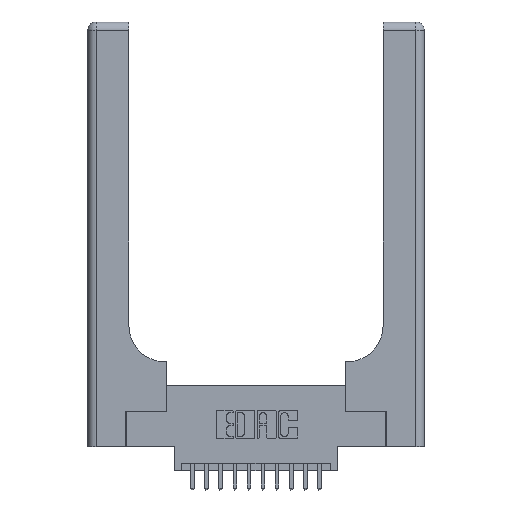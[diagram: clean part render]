
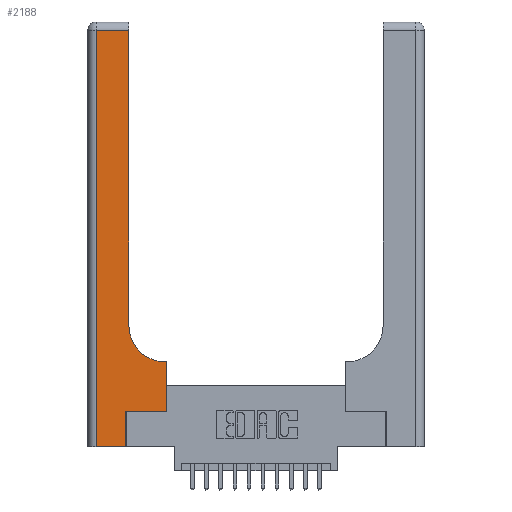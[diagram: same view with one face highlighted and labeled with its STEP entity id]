
A CAD part, top view. The second image highlights one B-rep face of the part: STEP entity #2188.
In plain terms, the highlighted planar face has unit normal (0, 0, 1).
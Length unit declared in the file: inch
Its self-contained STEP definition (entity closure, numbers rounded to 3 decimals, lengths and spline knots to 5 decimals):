
#117 = AXIS2_PLACEMENT_3D ( 'NONE', #14406, #6383, #15714 ) ;
#143 = EDGE_CURVE ( 'NONE', #3979, #8426, #5227, .T. ) ;
#165 = VERTEX_POINT ( 'NONE', #17461 ) ;
#1022 = ORIENTED_EDGE ( 'NONE', *, *, #143, .T. ) ;
#1057 = ORIENTED_EDGE ( 'NONE', *, *, #1328, .T. ) ;
#1191 = ORIENTED_EDGE ( 'NONE', *, *, #13848, .T. ) ;
#1328 = EDGE_CURVE ( 'NONE', #6525, #7529, #17280, .T. ) ;
#1577 = LINE ( 'NONE', #12074, #12004 ) ;
#1596 = CIRCLE ( 'NONE', #117, 0.25 ) ;
#1942 = EDGE_CURVE ( 'NONE', #3460, #11714, #5795, .T. ) ;
#2188 = ADVANCED_FACE ( 'NONE', ( #9169 ), #16580, .F. ) ;
#2648 = DIRECTION ( 'NONE',  ( 0., -1., 0. ) ) ;
#2666 = VERTEX_POINT ( 'NONE', #12107 ) ;
#2839 = EDGE_CURVE ( 'NONE', #2666, #165, #14156, .T. ) ;
#2860 = CARTESIAN_POINT ( 'NONE',  ( 0.06, 3., 0.37 ) ) ;
#3460 = VERTEX_POINT ( 'NONE', #4581 ) ;
#3979 = VERTEX_POINT ( 'NONE', #11305 ) ;
#3980 = CARTESIAN_POINT ( 'NONE',  ( 0.5585, 0.6, 0.37 ) ) ;
#4274 = VECTOR ( 'NONE', #10622, 39.37008 ) ;
#4581 = CARTESIAN_POINT ( 'NONE',  ( 0.2915, 0.85, 0.37 ) ) ;
#4816 = CARTESIAN_POINT ( 'NONE',  ( 0.2915, 3., 0.37 ) ) ;
#4951 = VECTOR ( 'NONE', #14915, 39.37008 ) ;
#5227 = LINE ( 'NONE', #9104, #12342 ) ;
#5795 = LINE ( 'NONE', #4816, #4951 ) ;
#5859 = EDGE_CURVE ( 'NONE', #10362, #3460, #1596, .T. ) ;
#6108 = CARTESIAN_POINT ( 'NONE',  ( 0.06, 0., 0.37 ) ) ;
#6243 = VECTOR ( 'NONE', #2648, 39.37008 ) ;
#6383 = DIRECTION ( 'NONE',  ( 0., 0., -1. ) ) ;
#6503 = LINE ( 'NONE', #16920, #16689 ) ;
#6525 = VERTEX_POINT ( 'NONE', #7737 ) ;
#6586 = LINE ( 'NONE', #15917, #7435 ) ;
#6600 = ORIENTED_EDGE ( 'NONE', *, *, #5859, .T. ) ;
#7007 = ORIENTED_EDGE ( 'NONE', *, *, #16245, .T. ) ;
#7385 = ORIENTED_EDGE ( 'NONE', *, *, #17091, .T. ) ;
#7435 = VECTOR ( 'NONE', #7964, 39.37008 ) ;
#7529 = VERTEX_POINT ( 'NONE', #6108 ) ;
#7737 = CARTESIAN_POINT ( 'NONE',  ( 0.06, 2.94, 0.37 ) ) ;
#7964 = DIRECTION ( 'NONE',  ( 1., 0., 0. ) ) ;
#8256 = ORIENTED_EDGE ( 'NONE', *, *, #1942, .T. ) ;
#8426 = VERTEX_POINT ( 'NONE', #3980 ) ;
#8581 = VECTOR ( 'NONE', #13203, 39.37008 ) ;
#8976 = DIRECTION ( 'NONE',  ( -1., 0., 0. ) ) ;
#9104 = CARTESIAN_POINT ( 'NONE',  ( 0.5585, 0.25, 0.37 ) ) ;
#9169 = FACE_OUTER_BOUND ( 'NONE', #12864, .T. ) ;
#9256 = ORIENTED_EDGE ( 'NONE', *, *, #13971, .T. ) ;
#10362 = VERTEX_POINT ( 'NONE', #13468 ) ;
#10622 = DIRECTION ( 'NONE',  ( 0., 1., 0. ) ) ;
#10803 = DIRECTION ( 'NONE',  ( -1., 0., 0. ) ) ;
#10840 = CARTESIAN_POINT ( 'NONE',  ( 0.269, 0., 0.37 ) ) ;
#11305 = CARTESIAN_POINT ( 'NONE',  ( 0.5585, 0.25, 0.37 ) ) ;
#11714 = VERTEX_POINT ( 'NONE', #13173 ) ;
#12004 = VECTOR ( 'NONE', #10803, 39.37008 ) ;
#12074 = CARTESIAN_POINT ( 'NONE',  ( 0.2915, 0.6, 0.37 ) ) ;
#12107 = CARTESIAN_POINT ( 'NONE',  ( 0.269, 0., 0.37 ) ) ;
#12342 = VECTOR ( 'NONE', #12434, 39.37008 ) ;
#12434 = DIRECTION ( 'NONE',  ( 0., 1., 0. ) ) ;
#12714 = ORIENTED_EDGE ( 'NONE', *, *, #2839, .T. ) ;
#12864 = EDGE_LOOP ( 'NONE', ( #8256, #7007, #1057, #1191, #12714, #7385, #1022, #9256, #6600 ) ) ;
#13173 = CARTESIAN_POINT ( 'NONE',  ( 0.2915, 2.94, 0.37 ) ) ;
#13203 = DIRECTION ( 'NONE',  ( 1., 0., 0. ) ) ;
#13468 = CARTESIAN_POINT ( 'NONE',  ( 0.5415, 0.6, 0.37 ) ) ;
#13848 = EDGE_CURVE ( 'NONE', #7529, #2666, #6586, .T. ) ;
#13971 = EDGE_CURVE ( 'NONE', #8426, #10362, #1577, .T. ) ;
#14156 = LINE ( 'NONE', #10840, #4274 ) ;
#14406 = CARTESIAN_POINT ( 'NONE',  ( 0.5415, 0.85, 0.37 ) ) ;
#14833 = LINE ( 'NONE', #15876, #8581 ) ;
#14915 = DIRECTION ( 'NONE',  ( 0., 1., 0. ) ) ;
#15714 = DIRECTION ( 'NONE',  ( 1., 0., 0. ) ) ;
#15876 = CARTESIAN_POINT ( 'NONE',  ( 0.269, 0.25, 0.37 ) ) ;
#15917 = CARTESIAN_POINT ( 'NONE',  ( 0., 0., 0.37 ) ) ;
#16245 = EDGE_CURVE ( 'NONE', #11714, #6525, #6503, .T. ) ;
#16384 = DIRECTION ( 'NONE',  ( -1., 0., 0. ) ) ;
#16401 = DIRECTION ( 'NONE',  ( 0., 0., -1. ) ) ;
#16452 = CARTESIAN_POINT ( 'NONE',  ( 0., 3., 0.37 ) ) ;
#16580 = PLANE ( 'NONE',  #16837 ) ;
#16689 = VECTOR ( 'NONE', #8976, 39.37008 ) ;
#16837 = AXIS2_PLACEMENT_3D ( 'NONE', #16452, #16401, #16384 ) ;
#16920 = CARTESIAN_POINT ( 'NONE',  ( 0., 2.94, 0.37 ) ) ;
#17091 = EDGE_CURVE ( 'NONE', #165, #3979, #14833, .T. ) ;
#17280 = LINE ( 'NONE', #2860, #6243 ) ;
#17461 = CARTESIAN_POINT ( 'NONE',  ( 0.269, 0.25, 0.37 ) ) ;
